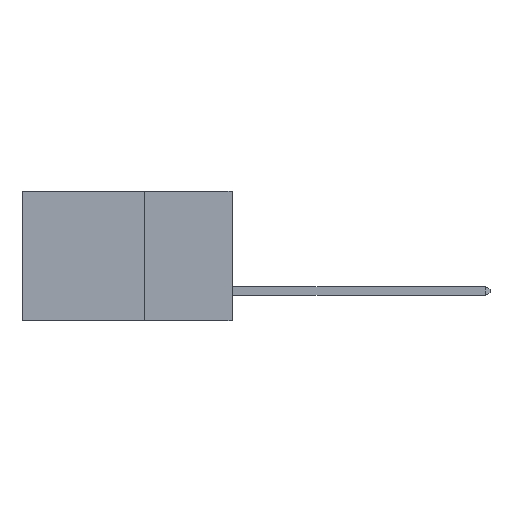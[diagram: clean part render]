
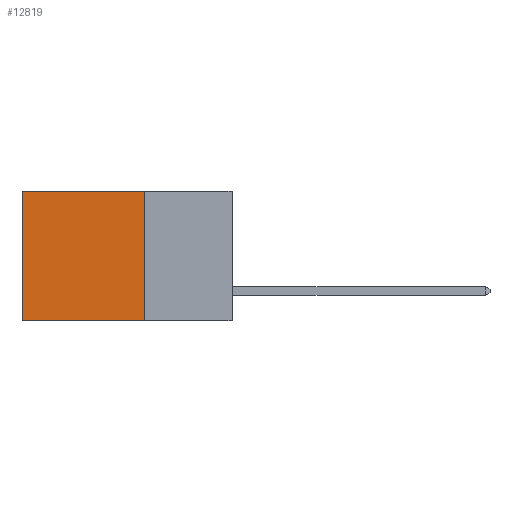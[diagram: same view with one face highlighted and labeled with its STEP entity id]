
A CAD part, left-side view. The second image highlights one B-rep face of the part: STEP entity #12819.
In plain terms, the highlighted planar face has unit normal (-1, 0, 0).
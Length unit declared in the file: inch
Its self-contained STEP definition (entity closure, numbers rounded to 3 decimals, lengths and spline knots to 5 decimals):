
#328 = PLANE ( 'NONE',  #3313 ) ;
#411 = ORIENTED_EDGE ( 'NONE', *, *, #12184, .T. ) ;
#1997 = DIRECTION ( 'NONE',  ( 0., 0., -1. ) ) ;
#2098 = CARTESIAN_POINT ( 'NONE',  ( 0.2875, 0.25, 0. ) ) ;
#3313 = AXIS2_PLACEMENT_3D ( 'NONE', #13674, #3752, #15272 ) ;
#3752 = DIRECTION ( 'NONE',  ( 1., 0., 0. ) ) ;
#3954 = FACE_OUTER_BOUND ( 'NONE', #21011, .T. ) ;
#3988 = VERTEX_POINT ( 'NONE', #14167 ) ;
#4351 = CARTESIAN_POINT ( 'NONE',  ( 0.2875, 0.6, 0. ) ) ;
#5436 = CARTESIAN_POINT ( 'NONE',  ( 0.2875, 0.25, -0.37 ) ) ;
#7030 = EDGE_CURVE ( 'NONE', #7305, #9428, #19631, .T. ) ;
#7194 = DIRECTION ( 'NONE',  ( 0., 1., 0. ) ) ;
#7305 = VERTEX_POINT ( 'NONE', #11084 ) ;
#7962 = LINE ( 'NONE', #4351, #20663 ) ;
#8047 = CARTESIAN_POINT ( 'NONE',  ( 0.2875, 0.6, -0.37 ) ) ;
#8101 = CARTESIAN_POINT ( 'NONE',  ( 0.2875, 0.25, 0. ) ) ;
#8946 = VECTOR ( 'NONE', #1997, 39.37008 ) ;
#9226 = VECTOR ( 'NONE', #13696, 39.37008 ) ;
#9428 = VERTEX_POINT ( 'NONE', #8047 ) ;
#11084 = CARTESIAN_POINT ( 'NONE',  ( 0.2875, 0.25, -0.37 ) ) ;
#11718 = ORIENTED_EDGE ( 'NONE', *, *, #7030, .F. ) ;
#12184 = EDGE_CURVE ( 'NONE', #15740, #3988, #20912, .T. ) ;
#12796 = EDGE_CURVE ( 'NONE', #15740, #7305, #13311, .T. ) ;
#12819 = ADVANCED_FACE ( 'NONE', ( #3954 ), #328, .F. ) ;
#13311 = LINE ( 'NONE', #16754, #8946 ) ;
#13674 = CARTESIAN_POINT ( 'NONE',  ( 0.2875, 0.25, 0. ) ) ;
#13696 = DIRECTION ( 'NONE',  ( 0., 1., 0. ) ) ;
#14167 = CARTESIAN_POINT ( 'NONE',  ( 0.2875, 0.6, 0. ) ) ;
#14263 = DIRECTION ( 'NONE',  ( 0., 0., -1. ) ) ;
#15272 = DIRECTION ( 'NONE',  ( 0., 0., -1. ) ) ;
#15514 = VECTOR ( 'NONE', #7194, 39.37008 ) ;
#15740 = VERTEX_POINT ( 'NONE', #8101 ) ;
#16754 = CARTESIAN_POINT ( 'NONE',  ( 0.2875, 0.25, 0. ) ) ;
#19346 = EDGE_CURVE ( 'NONE', #3988, #9428, #7962, .T. ) ;
#19631 = LINE ( 'NONE', #5436, #15514 ) ;
#20459 = ORIENTED_EDGE ( 'NONE', *, *, #19346, .T. ) ;
#20663 = VECTOR ( 'NONE', #14263, 39.37008 ) ;
#20912 = LINE ( 'NONE', #2098, #9226 ) ;
#20936 = ORIENTED_EDGE ( 'NONE', *, *, #12796, .F. ) ;
#21011 = EDGE_LOOP ( 'NONE', ( #20459, #11718, #20936, #411 ) ) ;
